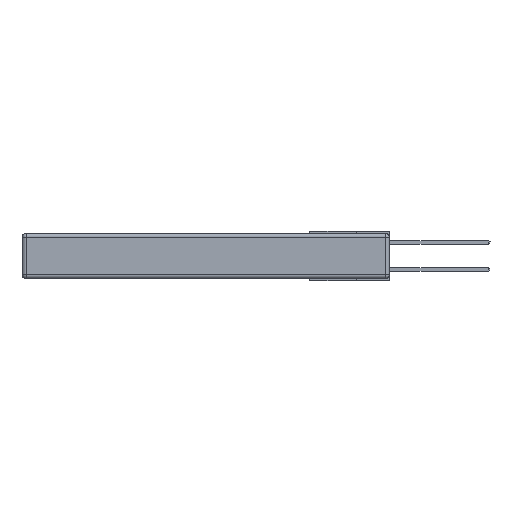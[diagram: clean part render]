
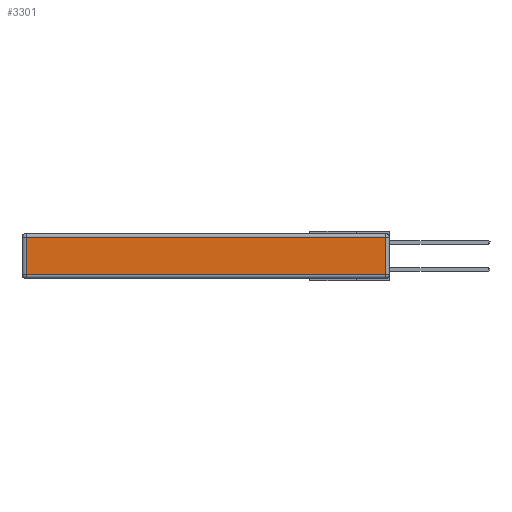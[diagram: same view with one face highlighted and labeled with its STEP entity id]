
A CAD part, left-side view. The second image highlights one B-rep face of the part: STEP entity #3301.
In plain terms, the highlighted planar face has unit normal (-1, 0, 0).
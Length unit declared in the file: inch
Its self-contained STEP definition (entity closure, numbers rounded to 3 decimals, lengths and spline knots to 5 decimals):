
#239 = LINE ( 'NONE', #2179, #16619 ) ;
#406 = LINE ( 'NONE', #26812, #18771 ) ;
#2179 = CARTESIAN_POINT ( 'NONE',  ( 0., 2.72, -0.343 ) ) ;
#2588 = DIRECTION ( 'NONE',  ( 0., 1., 0. ) ) ;
#3070 = ORIENTED_EDGE ( 'NONE', *, *, #25344, .T. ) ;
#3301 = ADVANCED_FACE ( 'NONE', ( #5770 ), #26776, .T. ) ;
#4502 = DIRECTION ( 'NONE',  ( 0., 0., -1. ) ) ;
#5470 = VERTEX_POINT ( 'NONE', #21294 ) ;
#5770 = FACE_OUTER_BOUND ( 'NONE', #9550, .T. ) ;
#6526 = CARTESIAN_POINT ( 'NONE',  ( 0., 2.75, -0.03 ) ) ;
#7322 = LINE ( 'NONE', #6526, #14362 ) ;
#8049 = CARTESIAN_POINT ( 'NONE',  ( 0., 0.03, -0.343 ) ) ;
#8736 = VECTOR ( 'NONE', #14312, 39.37008 ) ;
#9550 = EDGE_LOOP ( 'NONE', ( #19716, #15569, #3070, #15767 ) ) ;
#10627 = EDGE_CURVE ( 'NONE', #5470, #17806, #22030, .T. ) ;
#11914 = DIRECTION ( 'NONE',  ( 0., 0., 1. ) ) ;
#12201 = AXIS2_PLACEMENT_3D ( 'NONE', #24627, #16192, #11914 ) ;
#13378 = CARTESIAN_POINT ( 'NONE',  ( 0., 2.72, -0.313 ) ) ;
#14312 = DIRECTION ( 'NONE',  ( 0., 0., 1. ) ) ;
#14362 = VECTOR ( 'NONE', #2588, 39.37008 ) ;
#15437 = CARTESIAN_POINT ( 'NONE',  ( 0., 2.72, -0.03 ) ) ;
#15569 = ORIENTED_EDGE ( 'NONE', *, *, #10627, .T. ) ;
#15767 = ORIENTED_EDGE ( 'NONE', *, *, #23967, .T. ) ;
#16093 = VERTEX_POINT ( 'NONE', #15437 ) ;
#16192 = DIRECTION ( 'NONE',  ( -1., 0., 0. ) ) ;
#16619 = VECTOR ( 'NONE', #4502, 39.37008 ) ;
#17527 = EDGE_CURVE ( 'NONE', #25151, #5470, #406, .T. ) ;
#17806 = VERTEX_POINT ( 'NONE', #19548 ) ;
#18771 = VECTOR ( 'NONE', #22821, 39.37008 ) ;
#19548 = CARTESIAN_POINT ( 'NONE',  ( 0., 0.03, -0.03 ) ) ;
#19716 = ORIENTED_EDGE ( 'NONE', *, *, #17527, .T. ) ;
#21294 = CARTESIAN_POINT ( 'NONE',  ( 0., 0.03, -0.313 ) ) ;
#22030 = LINE ( 'NONE', #8049, #8736 ) ;
#22821 = DIRECTION ( 'NONE',  ( 0., -1., 0. ) ) ;
#23967 = EDGE_CURVE ( 'NONE', #16093, #25151, #239, .T. ) ;
#24627 = CARTESIAN_POINT ( 'NONE',  ( 0., 0., -0.343 ) ) ;
#25151 = VERTEX_POINT ( 'NONE', #13378 ) ;
#25344 = EDGE_CURVE ( 'NONE', #17806, #16093, #7322, .T. ) ;
#26776 = PLANE ( 'NONE',  #12201 ) ;
#26812 = CARTESIAN_POINT ( 'NONE',  ( 0., 0., -0.313 ) ) ;
